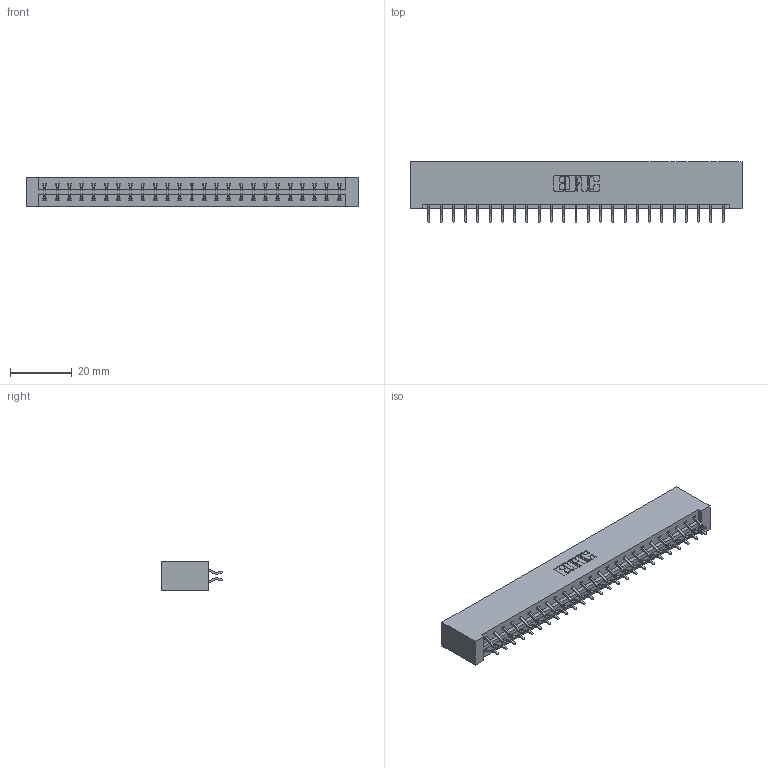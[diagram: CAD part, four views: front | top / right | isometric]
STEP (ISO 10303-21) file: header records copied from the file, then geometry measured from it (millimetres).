
FILE_DESCRIPTION (( 'STEP AP203' ), '1' );
FILE_NAME ('333-050-556-201.STEP', '2018-08-04T01:18:25', ( '' ), ( '' ), 'SwSTEP 2.0', 'SolidWorks 2016', '' );
FILE_SCHEMA (( 'CONFIG_CONTROL_DESIGN' ));
Length unit declared in the file: inch
Products named in the file (3): 333 Part_Lugless; 345-292-001_556 Tail; 333-050-556-201
Assembly tree (51 placements, depth 2):
  333-050-556-201
    333 Part_Lugless
    345-292-001_556 Tail  x50
Bounding box: 107.31 x 19.57 x 9.4 mm (x, y, z)
Volume: 11427.5 mm3; surface area: 13302.5 mm2
Topology: 51 solids, 51 shells, 3006 faces, 8937 edges, 5890 vertices
Faces by surface type: plane 2066, cylinder 940
Entity records: 18225 total; most frequent: CARTESIAN_POINT 3054, ORIENTED_EDGE 2978, DIRECTION 2621, EDGE_CURVE 1489, LINE 1361, VECTOR 1361, VERTEX_POINT 990, AXIS2_PLACEMENT_3D 630
